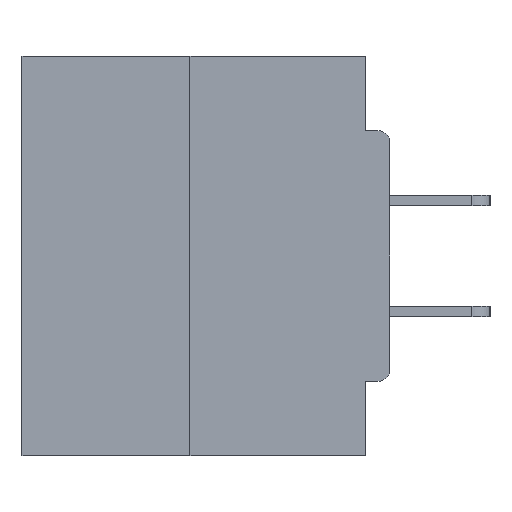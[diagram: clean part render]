
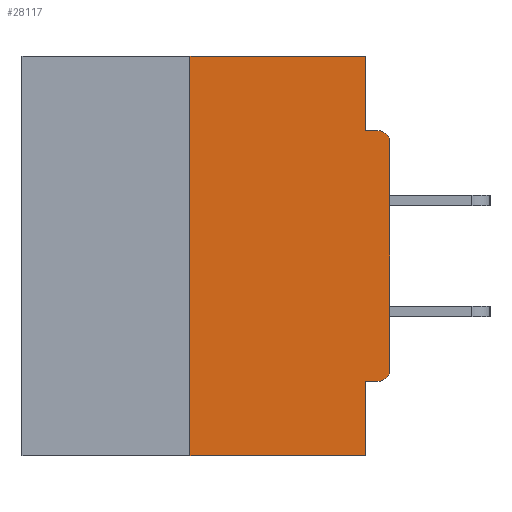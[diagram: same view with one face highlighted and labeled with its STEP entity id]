
A CAD part, left-side view. The second image highlights one B-rep face of the part: STEP entity #28117.
In plain terms, the highlighted planar face has unit normal (-1, 0, 0).
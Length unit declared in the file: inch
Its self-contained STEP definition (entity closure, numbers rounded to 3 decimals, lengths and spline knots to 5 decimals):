
#128 = CIRCLE ( 'NONE', #7507, 0.015 ) ;
#794 = EDGE_CURVE ( 'NONE', #7720, #7523, #128, .T. ) ;
#1731 = FACE_OUTER_BOUND ( 'NONE', #36162, .T. ) ;
#2133 = DIRECTION ( 'NONE',  ( 0., 0., -1. ) ) ;
#2292 = CARTESIAN_POINT ( 'NONE',  ( 0., 0.031, 0. ) ) ;
#2394 = LINE ( 'NONE', #36882, #9571 ) ;
#2525 = CARTESIAN_POINT ( 'NONE',  ( 0., 0.031, -0.5 ) ) ;
#2742 = CARTESIAN_POINT ( 'NONE',  ( 0., 0., -0.1085 ) ) ;
#2752 = LINE ( 'NONE', #29530, #13132 ) ;
#2962 = EDGE_CURVE ( 'NONE', #10258, #3191, #13430, .T. ) ;
#3001 = VECTOR ( 'NONE', #8117, 39.37008 ) ;
#3191 = VERTEX_POINT ( 'NONE', #6255 ) ;
#3553 = EDGE_CURVE ( 'NONE', #15952, #7720, #2394, .T. ) ;
#3758 = LINE ( 'NONE', #6833, #17371 ) ;
#3960 = DIRECTION ( 'NONE',  ( 0., 1., 0. ) ) ;
#4494 = ORIENTED_EDGE ( 'NONE', *, *, #2962, .F. ) ;
#5250 = LINE ( 'NONE', #11585, #3001 ) ;
#5439 = EDGE_CURVE ( 'NONE', #19473, #15952, #28933, .T. ) ;
#6255 = CARTESIAN_POINT ( 'NONE',  ( 0., 0.25, 0. ) ) ;
#6432 = VERTEX_POINT ( 'NONE', #19035 ) ;
#6833 = CARTESIAN_POINT ( 'NONE',  ( 0., 0., -0.4065 ) ) ;
#7507 = AXIS2_PLACEMENT_3D ( 'NONE', #23580, #23400, #11835 ) ;
#7523 = VERTEX_POINT ( 'NONE', #25876 ) ;
#7560 = ORIENTED_EDGE ( 'NONE', *, *, #19107, .F. ) ;
#7720 = VERTEX_POINT ( 'NONE', #2742 ) ;
#8117 = DIRECTION ( 'NONE',  ( 0., -1., 0. ) ) ;
#8160 = DIRECTION ( 'NONE',  ( 0., 0., 1. ) ) ;
#8606 = DIRECTION ( 'NONE',  ( 0., 0., -1. ) ) ;
#9571 = VECTOR ( 'NONE', #8160, 39.37008 ) ;
#10258 = VERTEX_POINT ( 'NONE', #26838 ) ;
#10635 = AXIS2_PLACEMENT_3D ( 'NONE', #16181, #22149, #34139 ) ;
#11585 = CARTESIAN_POINT ( 'NONE',  ( 0., 0.46, 0. ) ) ;
#11835 = DIRECTION ( 'NONE',  ( 0., 0., -1. ) ) ;
#12019 = ORIENTED_EDGE ( 'NONE', *, *, #35451, .F. ) ;
#12507 = EDGE_CURVE ( 'NONE', #6432, #37448, #14462, .T. ) ;
#12650 = ORIENTED_EDGE ( 'NONE', *, *, #34523, .F. ) ;
#13132 = VECTOR ( 'NONE', #14514, 39.37008 ) ;
#13430 = LINE ( 'NONE', #25162, #23029 ) ;
#13501 = PLANE ( 'NONE',  #10635 ) ;
#13954 = ORIENTED_EDGE ( 'NONE', *, *, #3553, .T. ) ;
#14209 = CARTESIAN_POINT ( 'NONE',  ( 0., 0., -0.0935 ) ) ;
#14462 = LINE ( 'NONE', #2525, #16435 ) ;
#14514 = DIRECTION ( 'NONE',  ( 0., -1., 0. ) ) ;
#14596 = DIRECTION ( 'NONE',  ( -1., 0., 0. ) ) ;
#15594 = EDGE_CURVE ( 'NONE', #25313, #28078, #37154, .T. ) ;
#15631 = ORIENTED_EDGE ( 'NONE', *, *, #5439, .T. ) ;
#15952 = VERTEX_POINT ( 'NONE', #30320 ) ;
#16181 = CARTESIAN_POINT ( 'NONE',  ( 0., 0.46, 0. ) ) ;
#16435 = VECTOR ( 'NONE', #2133, 39.37008 ) ;
#17371 = VECTOR ( 'NONE', #3960, 39.37008 ) ;
#18686 = ORIENTED_EDGE ( 'NONE', *, *, #29156, .T. ) ;
#18981 = ORIENTED_EDGE ( 'NONE', *, *, #12507, .F. ) ;
#19035 = CARTESIAN_POINT ( 'NONE',  ( 0., 0.031, -0.4065 ) ) ;
#19107 = EDGE_CURVE ( 'NONE', #3191, #25313, #5250, .T. ) ;
#19473 = VERTEX_POINT ( 'NONE', #37745 ) ;
#20914 = VECTOR ( 'NONE', #25381, 39.37008 ) ;
#22149 = DIRECTION ( 'NONE',  ( 1., 0., 0. ) ) ;
#22834 = DIRECTION ( 'NONE',  ( 0., 0., 1. ) ) ;
#22970 = VECTOR ( 'NONE', #37132, 39.37008 ) ;
#23029 = VECTOR ( 'NONE', #22834, 39.37008 ) ;
#23400 = DIRECTION ( 'NONE',  ( -1., 0., 0. ) ) ;
#23580 = CARTESIAN_POINT ( 'NONE',  ( 0., 0.015, -0.1085 ) ) ;
#24476 = CARTESIAN_POINT ( 'NONE',  ( 0., 0.031, -0.0935 ) ) ;
#25162 = CARTESIAN_POINT ( 'NONE',  ( 0., 0.25, 0. ) ) ;
#25313 = VERTEX_POINT ( 'NONE', #32320 ) ;
#25381 = DIRECTION ( 'NONE',  ( 0., 0., -1. ) ) ;
#25876 = CARTESIAN_POINT ( 'NONE',  ( 0., 0.015, -0.0935 ) ) ;
#26838 = CARTESIAN_POINT ( 'NONE',  ( 0., 0.25, -0.5 ) ) ;
#28078 = VERTEX_POINT ( 'NONE', #24476 ) ;
#28117 = ADVANCED_FACE ( 'NONE', ( #1731 ), #13501, .F. ) ;
#28831 = ORIENTED_EDGE ( 'NONE', *, *, #794, .T. ) ;
#28853 = LINE ( 'NONE', #14209, #22970 ) ;
#28933 = CIRCLE ( 'NONE', #37552, 0.015 ) ;
#29156 = EDGE_CURVE ( 'NONE', #10258, #37448, #2752, .T. ) ;
#29530 = CARTESIAN_POINT ( 'NONE',  ( 0., 0.46, -0.5 ) ) ;
#30320 = CARTESIAN_POINT ( 'NONE',  ( 0., 0., -0.3915 ) ) ;
#31779 = CARTESIAN_POINT ( 'NONE',  ( 0., 0.015, -0.3915 ) ) ;
#32320 = CARTESIAN_POINT ( 'NONE',  ( 0., 0.031, 0. ) ) ;
#33033 = CARTESIAN_POINT ( 'NONE',  ( 0., 0.031, -0.5 ) ) ;
#34139 = DIRECTION ( 'NONE',  ( 0., 0., -1. ) ) ;
#34523 = EDGE_CURVE ( 'NONE', #19473, #6432, #3758, .T. ) ;
#35451 = EDGE_CURVE ( 'NONE', #28078, #7523, #28853, .T. ) ;
#36162 = EDGE_LOOP ( 'NONE', ( #7560, #4494, #18686, #18981, #12650, #15631, #13954, #28831, #12019, #36895 ) ) ;
#36882 = CARTESIAN_POINT ( 'NONE',  ( 0., 0., 0. ) ) ;
#36895 = ORIENTED_EDGE ( 'NONE', *, *, #15594, .F. ) ;
#37132 = DIRECTION ( 'NONE',  ( 0., -1., 0. ) ) ;
#37154 = LINE ( 'NONE', #2292, #20914 ) ;
#37448 = VERTEX_POINT ( 'NONE', #33033 ) ;
#37552 = AXIS2_PLACEMENT_3D ( 'NONE', #31779, #14596, #8606 ) ;
#37745 = CARTESIAN_POINT ( 'NONE',  ( 0., 0.015, -0.4065 ) ) ;
